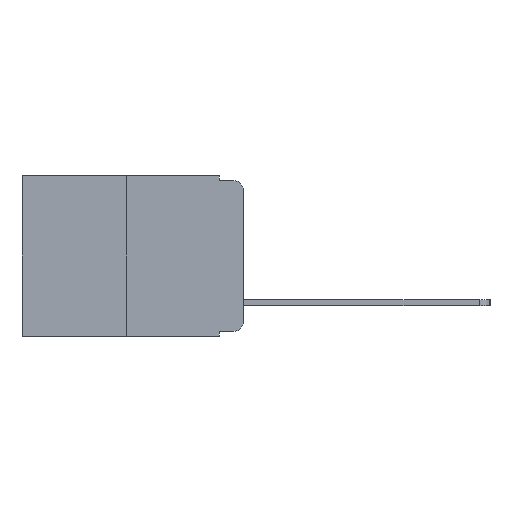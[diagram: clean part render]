
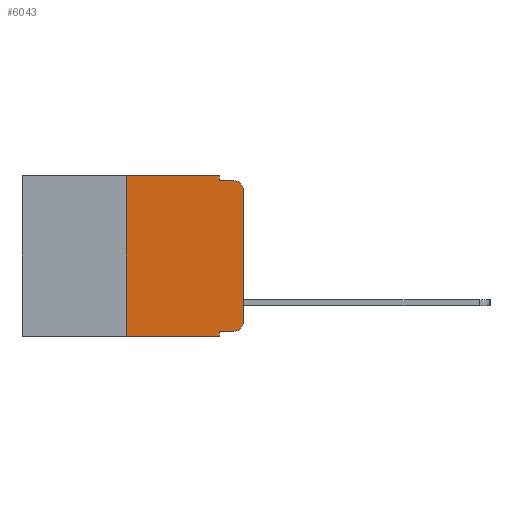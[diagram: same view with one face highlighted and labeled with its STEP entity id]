
A CAD part, left-side view. The second image highlights one B-rep face of the part: STEP entity #6043.
In plain terms, the highlighted planar face has unit normal (-1, 0, 0).
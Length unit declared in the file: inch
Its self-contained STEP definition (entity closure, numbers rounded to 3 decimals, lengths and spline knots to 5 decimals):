
#513 = ORIENTED_EDGE ( 'NONE', *, *, #11189, .T. ) ;
#548 = PLANE ( 'NONE',  #3882 ) ;
#631 = CARTESIAN_POINT ( 'NONE',  ( 0., 0.25, -0.343 ) ) ;
#637 = LINE ( 'NONE', #10054, #9718 ) ;
#687 = ORIENTED_EDGE ( 'NONE', *, *, #3536, .F. ) ;
#734 = CARTESIAN_POINT ( 'NONE',  ( 0., 0., -0.313 ) ) ;
#839 = CARTESIAN_POINT ( 'NONE',  ( 0., 0.051, 0. ) ) ;
#926 = ORIENTED_EDGE ( 'NONE', *, *, #7235, .T. ) ;
#1104 = ORIENTED_EDGE ( 'NONE', *, *, #3611, .T. ) ;
#1149 = ORIENTED_EDGE ( 'NONE', *, *, #2920, .F. ) ;
#1384 = ORIENTED_EDGE ( 'NONE', *, *, #6067, .F. ) ;
#1599 = LINE ( 'NONE', #3516, #8357 ) ;
#2048 = EDGE_CURVE ( 'NONE', #9745, #4086, #4526, .T. ) ;
#2130 = LINE ( 'NONE', #839, #11118 ) ;
#2240 = DIRECTION ( 'NONE',  ( -1., 0., 0. ) ) ;
#2340 = ORIENTED_EDGE ( 'NONE', *, *, #6651, .F. ) ;
#2585 = DIRECTION ( 'NONE',  ( 1., 0., 0. ) ) ;
#2624 = AXIS2_PLACEMENT_3D ( 'NONE', #7501, #2240, #8334 ) ;
#2666 = VERTEX_POINT ( 'NONE', #10752 ) ;
#2765 = ORIENTED_EDGE ( 'NONE', *, *, #2048, .T. ) ;
#2856 = DIRECTION ( 'NONE',  ( 0., 0., -1. ) ) ;
#2920 = EDGE_CURVE ( 'NONE', #5277, #4086, #2130, .T. ) ;
#3011 = EDGE_CURVE ( 'NONE', #5277, #7873, #5462, .T. ) ;
#3340 = DIRECTION ( 'NONE',  ( 0., 0., -1. ) ) ;
#3516 = CARTESIAN_POINT ( 'NONE',  ( 0., 0.051, -0.01 ) ) ;
#3536 = EDGE_CURVE ( 'NONE', #9745, #9597, #9134, .T. ) ;
#3611 = EDGE_CURVE ( 'NONE', #7873, #6184, #10493, .T. ) ;
#3621 = DIRECTION ( 'NONE',  ( 0., -1., 0. ) ) ;
#3842 = VECTOR ( 'NONE', #3621, 39.37008 ) ;
#3870 = VECTOR ( 'NONE', #9680, 39.37008 ) ;
#3882 = AXIS2_PLACEMENT_3D ( 'NONE', #7791, #2585, #8608 ) ;
#3966 = CARTESIAN_POINT ( 'NONE',  ( 0., 0., -0.03 ) ) ;
#4052 = EDGE_CURVE ( 'NONE', #9597, #5328, #8382, .T. ) ;
#4086 = VERTEX_POINT ( 'NONE', #4539 ) ;
#4521 = VERTEX_POINT ( 'NONE', #8487 ) ;
#4526 = LINE ( 'NONE', #6135, #10856 ) ;
#4539 = CARTESIAN_POINT ( 'NONE',  ( 0., 0.051, -0.343 ) ) ;
#5049 = CARTESIAN_POINT ( 'NONE',  ( 0., 0.25, 0. ) ) ;
#5253 = CIRCLE ( 'NONE', #2624, 0.02 ) ;
#5277 = VERTEX_POINT ( 'NONE', #8617 ) ;
#5328 = VERTEX_POINT ( 'NONE', #7836 ) ;
#5405 = CARTESIAN_POINT ( 'NONE',  ( 0., 0.02, -0.313 ) ) ;
#5462 = LINE ( 'NONE', #8125, #9907 ) ;
#5860 = DIRECTION ( 'NONE',  ( 0., -1., 0. ) ) ;
#6043 = ADVANCED_FACE ( 'NONE', ( #8614 ), #548, .F. ) ;
#6067 = EDGE_CURVE ( 'NONE', #4521, #2666, #1599, .T. ) ;
#6135 = CARTESIAN_POINT ( 'NONE',  ( 0., 0.473, -0.343 ) ) ;
#6184 = VERTEX_POINT ( 'NONE', #734 ) ;
#6275 = DIRECTION ( 'NONE',  ( 0., 0., -1. ) ) ;
#6651 = EDGE_CURVE ( 'NONE', #5328, #4521, #637, .T. ) ;
#6960 = VECTOR ( 'NONE', #11048, 39.37008 ) ;
#7182 = ORIENTED_EDGE ( 'NONE', *, *, #3011, .T. ) ;
#7235 = EDGE_CURVE ( 'NONE', #9433, #2666, #5253, .T. ) ;
#7501 = CARTESIAN_POINT ( 'NONE',  ( 0., 0.02, -0.03 ) ) ;
#7567 = ORIENTED_EDGE ( 'NONE', *, *, #4052, .F. ) ;
#7791 = CARTESIAN_POINT ( 'NONE',  ( 0., 0.473, 0. ) ) ;
#7835 = CARTESIAN_POINT ( 'NONE',  ( 0., 0.25, 0. ) ) ;
#7836 = CARTESIAN_POINT ( 'NONE',  ( 0., 0.051, 0. ) ) ;
#7873 = VERTEX_POINT ( 'NONE', #8470 ) ;
#8125 = CARTESIAN_POINT ( 'NONE',  ( 0., 0.051, -0.333 ) ) ;
#8334 = DIRECTION ( 'NONE',  ( 0., 0., -1. ) ) ;
#8357 = VECTOR ( 'NONE', #8640, 39.37008 ) ;
#8382 = LINE ( 'NONE', #11039, #3842 ) ;
#8470 = CARTESIAN_POINT ( 'NONE',  ( 0., 0.02, -0.333 ) ) ;
#8487 = CARTESIAN_POINT ( 'NONE',  ( 0., 0.051, -0.01 ) ) ;
#8543 = EDGE_LOOP ( 'NONE', ( #513, #926, #1384, #2340, #7567, #687, #2765, #1149, #7182, #1104 ) ) ;
#8608 = DIRECTION ( 'NONE',  ( 0., 0., -1. ) ) ;
#8614 = FACE_OUTER_BOUND ( 'NONE', #8543, .T. ) ;
#8617 = CARTESIAN_POINT ( 'NONE',  ( 0., 0.051, -0.333 ) ) ;
#8640 = DIRECTION ( 'NONE',  ( 0., -1., 0. ) ) ;
#8838 = AXIS2_PLACEMENT_3D ( 'NONE', #5405, #11149, #6275 ) ;
#8873 = CARTESIAN_POINT ( 'NONE',  ( 0., 0., 0. ) ) ;
#9134 = LINE ( 'NONE', #7835, #6960 ) ;
#9433 = VERTEX_POINT ( 'NONE', #3966 ) ;
#9597 = VERTEX_POINT ( 'NONE', #5049 ) ;
#9680 = DIRECTION ( 'NONE',  ( 0., 0., 1. ) ) ;
#9718 = VECTOR ( 'NONE', #3340, 39.37008 ) ;
#9745 = VERTEX_POINT ( 'NONE', #631 ) ;
#9907 = VECTOR ( 'NONE', #10479, 39.37008 ) ;
#10054 = CARTESIAN_POINT ( 'NONE',  ( 0., 0.051, 0. ) ) ;
#10280 = LINE ( 'NONE', #8873, #3870 ) ;
#10479 = DIRECTION ( 'NONE',  ( 0., -1., 0. ) ) ;
#10493 = CIRCLE ( 'NONE', #8838, 0.02 ) ;
#10752 = CARTESIAN_POINT ( 'NONE',  ( 0., 0.02, -0.01 ) ) ;
#10856 = VECTOR ( 'NONE', #5860, 39.37008 ) ;
#11039 = CARTESIAN_POINT ( 'NONE',  ( 0., 0.473, 0. ) ) ;
#11048 = DIRECTION ( 'NONE',  ( 0., 0., 1. ) ) ;
#11118 = VECTOR ( 'NONE', #2856, 39.37008 ) ;
#11149 = DIRECTION ( 'NONE',  ( -1., 0., 0. ) ) ;
#11189 = EDGE_CURVE ( 'NONE', #6184, #9433, #10280, .T. ) ;
